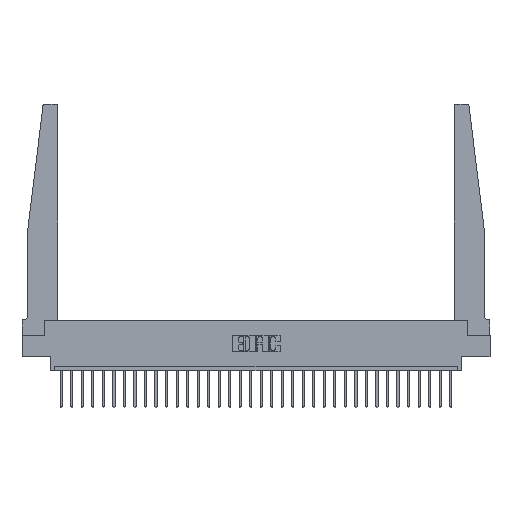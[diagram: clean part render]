
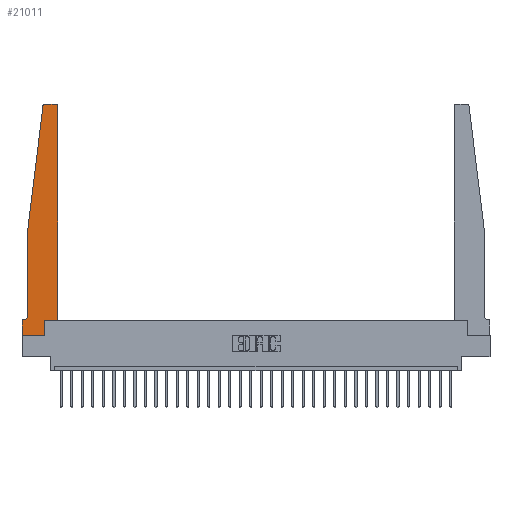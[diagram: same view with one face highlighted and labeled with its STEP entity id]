
A CAD part, top view. The second image highlights one B-rep face of the part: STEP entity #21011.
In plain terms, the highlighted planar face has unit normal (0, 0, 1).
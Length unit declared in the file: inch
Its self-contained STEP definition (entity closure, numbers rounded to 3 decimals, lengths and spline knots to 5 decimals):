
#529 = CARTESIAN_POINT ( 'NONE',  ( 0.015, 0.1875, 0.37 ) ) ;
#1069 = EDGE_CURVE ( 'NONE', #13363, #4208, #18889, .T. ) ;
#1365 = CARTESIAN_POINT ( 'NONE',  ( 0.065, 1.25, 0.37 ) ) ;
#1729 = ORIENTED_EDGE ( 'NONE', *, *, #20655, .T. ) ;
#2079 = EDGE_CURVE ( 'NONE', #8273, #14661, #13761, .T. ) ;
#2356 = EDGE_CURVE ( 'NONE', #4208, #14819, #29079, .T. ) ;
#2409 = CARTESIAN_POINT ( 'NONE',  ( 0.25, 2.75, 0.37 ) ) ;
#2510 = VERTEX_POINT ( 'NONE', #15670 ) ;
#2868 = CARTESIAN_POINT ( 'NONE',  ( 0.2605, 0.18, 0.37 ) ) ;
#2871 = EDGE_CURVE ( 'NONE', #2510, #8273, #11028, .T. ) ;
#3430 = CARTESIAN_POINT ( 'NONE',  ( 0.2605, 0.18, 0.37 ) ) ;
#3940 = VERTEX_POINT ( 'NONE', #15506 ) ;
#4171 = PLANE ( 'NONE',  #23163 ) ;
#4208 = VERTEX_POINT ( 'NONE', #24716 ) ;
#4264 = ORIENTED_EDGE ( 'NONE', *, *, #21400, .T. ) ;
#4683 = DIRECTION ( 'NONE',  ( 1., 0., 0. ) ) ;
#4842 = LINE ( 'NONE', #25095, #26031 ) ;
#6254 = ORIENTED_EDGE ( 'NONE', *, *, #2871, .T. ) ;
#6404 = CARTESIAN_POINT ( 'NONE',  ( 0.425, 0.18, 0.37 ) ) ;
#6991 = CARTESIAN_POINT ( 'NONE',  ( 0., 0., 0.37 ) ) ;
#7999 = VERTEX_POINT ( 'NONE', #13879 ) ;
#8151 = ORIENTED_EDGE ( 'NONE', *, *, #14392, .T. ) ;
#8231 = ORIENTED_EDGE ( 'NONE', *, *, #27320, .T. ) ;
#8273 = VERTEX_POINT ( 'NONE', #21449 ) ;
#8526 = DIRECTION ( 'NONE',  ( 1., 0., 0. ) ) ;
#8831 = DIRECTION ( 'NONE',  ( 0., 0., -1. ) ) ;
#8919 = DIRECTION ( 'NONE',  ( 0., 1., 0. ) ) ;
#9029 = LINE ( 'NONE', #13642, #20090 ) ;
#9131 = LINE ( 'NONE', #2409, #26739 ) ;
#9288 = DIRECTION ( 'NONE',  ( 1., 0., 0. ) ) ;
#9385 = EDGE_LOOP ( 'NONE', ( #18421, #18578, #18105, #4264, #1729, #8151, #6254, #10678, #28847, #8231, #16057, #27052 ) ) ;
#10360 = VECTOR ( 'NONE', #22478, 39.37008 ) ;
#10678 = ORIENTED_EDGE ( 'NONE', *, *, #2079, .T. ) ;
#10771 = CARTESIAN_POINT ( 'NONE',  ( 0.27653, 2.75, 0.37 ) ) ;
#11028 = LINE ( 'NONE', #6991, #10360 ) ;
#11058 = CIRCLE ( 'NONE', #20541, 0.03 ) ;
#11475 = DIRECTION ( 'NONE',  ( 1., 0., 0. ) ) ;
#11531 = CARTESIAN_POINT ( 'NONE',  ( 0., 0., 0.37 ) ) ;
#12004 = VERTEX_POINT ( 'NONE', #2868 ) ;
#12696 = CIRCLE ( 'NONE', #29338, 0.05 ) ;
#13363 = VERTEX_POINT ( 'NONE', #10771 ) ;
#13477 = CARTESIAN_POINT ( 'NONE',  ( 0.065, 1.25, 0.37 ) ) ;
#13596 = DIRECTION ( 'NONE',  ( -1., 0., 0. ) ) ;
#13642 = CARTESIAN_POINT ( 'NONE',  ( 0.425, 0.18, 0.37 ) ) ;
#13668 = AXIS2_PLACEMENT_3D ( 'NONE', #28775, #19827, #8526 ) ;
#13761 = LINE ( 'NONE', #11531, #15641 ) ;
#13879 = CARTESIAN_POINT ( 'NONE',  ( 0.065, 0.2375, 0.37 ) ) ;
#14392 = EDGE_CURVE ( 'NONE', #16540, #2510, #15750, .T. ) ;
#14661 = VERTEX_POINT ( 'NONE', #24045 ) ;
#14819 = VERTEX_POINT ( 'NONE', #13477 ) ;
#14903 = CARTESIAN_POINT ( 'NONE',  ( 0.425, 2.72, 0.37 ) ) ;
#14926 = DIRECTION ( 'NONE',  ( -0.122, -0.992, 0. ) ) ;
#15506 = CARTESIAN_POINT ( 'NONE',  ( 0.425, 0.18, 0.37 ) ) ;
#15641 = VECTOR ( 'NONE', #9288, 39.37008 ) ;
#15670 = CARTESIAN_POINT ( 'NONE',  ( 0., 0.1875, 0.37 ) ) ;
#15750 = LINE ( 'NONE', #27062, #21380 ) ;
#16057 = ORIENTED_EDGE ( 'NONE', *, *, #29140, .T. ) ;
#16239 = VECTOR ( 'NONE', #27239, 39.37008 ) ;
#16540 = VERTEX_POINT ( 'NONE', #529 ) ;
#17098 = EDGE_CURVE ( 'NONE', #20808, #21541, #11058, .T. ) ;
#17689 = VECTOR ( 'NONE', #14926, 39.37008 ) ;
#17995 = LINE ( 'NONE', #3430, #18164 ) ;
#18093 = DIRECTION ( 'NONE',  ( 0., 0., 1. ) ) ;
#18105 = ORIENTED_EDGE ( 'NONE', *, *, #2356, .T. ) ;
#18151 = LINE ( 'NONE', #6404, #16239 ) ;
#18164 = VECTOR ( 'NONE', #8919, 39.37008 ) ;
#18241 = DIRECTION ( 'NONE',  ( 0., -1., 0. ) ) ;
#18378 = CARTESIAN_POINT ( 'NONE',  ( 0.395, 2.72, 0.37 ) ) ;
#18421 = ORIENTED_EDGE ( 'NONE', *, *, #28267, .T. ) ;
#18578 = ORIENTED_EDGE ( 'NONE', *, *, #1069, .T. ) ;
#18889 = CIRCLE ( 'NONE', #13668, 0.03 ) ;
#19827 = DIRECTION ( 'NONE',  ( 0., 0., 1. ) ) ;
#20090 = VECTOR ( 'NONE', #20475, 39.37008 ) ;
#20096 = FACE_OUTER_BOUND ( 'NONE', #9385, .T. ) ;
#20133 = DIRECTION ( 'NONE',  ( -1., 0., 0. ) ) ;
#20475 = DIRECTION ( 'NONE',  ( 0., 1., 0. ) ) ;
#20541 = AXIS2_PLACEMENT_3D ( 'NONE', #18378, #18093, #4683 ) ;
#20655 = EDGE_CURVE ( 'NONE', #7999, #16540, #12696, .T. ) ;
#20808 = VERTEX_POINT ( 'NONE', #14903 ) ;
#21011 = ADVANCED_FACE ( 'NONE', ( #20096 ), #4171, .T. ) ;
#21380 = VECTOR ( 'NONE', #22731, 39.37008 ) ;
#21400 = EDGE_CURVE ( 'NONE', #14819, #7999, #4842, .T. ) ;
#21449 = CARTESIAN_POINT ( 'NONE',  ( 0., 0., 0.37 ) ) ;
#21541 = VERTEX_POINT ( 'NONE', #28215 ) ;
#22199 = DIRECTION ( 'NONE',  ( 0., 0., 1. ) ) ;
#22478 = DIRECTION ( 'NONE',  ( 0., -1., 0. ) ) ;
#22731 = DIRECTION ( 'NONE',  ( -1., 0., 0. ) ) ;
#23163 = AXIS2_PLACEMENT_3D ( 'NONE', #24870, #22199, #11475 ) ;
#24045 = CARTESIAN_POINT ( 'NONE',  ( 0.2605, 0., 0.37 ) ) ;
#24716 = CARTESIAN_POINT ( 'NONE',  ( 0.24675, 2.72367, 0.37 ) ) ;
#24870 = CARTESIAN_POINT ( 'NONE',  ( 0., 0.1875, 0.37 ) ) ;
#25095 = CARTESIAN_POINT ( 'NONE',  ( 0.065, 1.25, 0.37 ) ) ;
#25198 = CARTESIAN_POINT ( 'NONE',  ( 0.015, 0.2375, 0.37 ) ) ;
#26031 = VECTOR ( 'NONE', #18241, 39.37008 ) ;
#26739 = VECTOR ( 'NONE', #13596, 39.37008 ) ;
#27052 = ORIENTED_EDGE ( 'NONE', *, *, #17098, .T. ) ;
#27062 = CARTESIAN_POINT ( 'NONE',  ( 0.065, 0.1875, 0.37 ) ) ;
#27239 = DIRECTION ( 'NONE',  ( 1., 0., 0. ) ) ;
#27320 = EDGE_CURVE ( 'NONE', #12004, #3940, #18151, .T. ) ;
#28215 = CARTESIAN_POINT ( 'NONE',  ( 0.395, 2.75, 0.37 ) ) ;
#28267 = EDGE_CURVE ( 'NONE', #21541, #13363, #9131, .T. ) ;
#28478 = EDGE_CURVE ( 'NONE', #14661, #12004, #17995, .T. ) ;
#28775 = CARTESIAN_POINT ( 'NONE',  ( 0.27653, 2.72, 0.37 ) ) ;
#28847 = ORIENTED_EDGE ( 'NONE', *, *, #28478, .T. ) ;
#29079 = LINE ( 'NONE', #1365, #17689 ) ;
#29140 = EDGE_CURVE ( 'NONE', #3940, #20808, #9029, .T. ) ;
#29338 = AXIS2_PLACEMENT_3D ( 'NONE', #25198, #8831, #20133 ) ;
